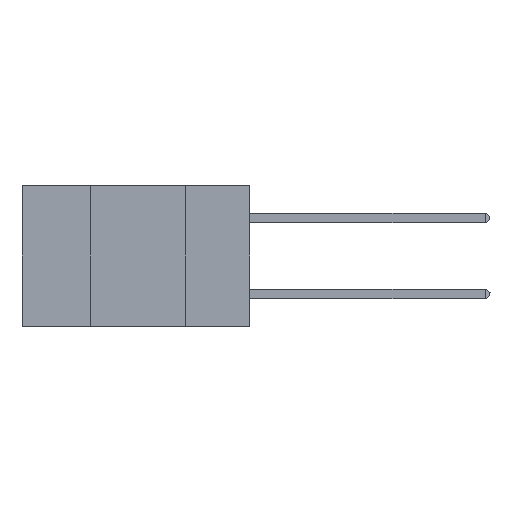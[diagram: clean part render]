
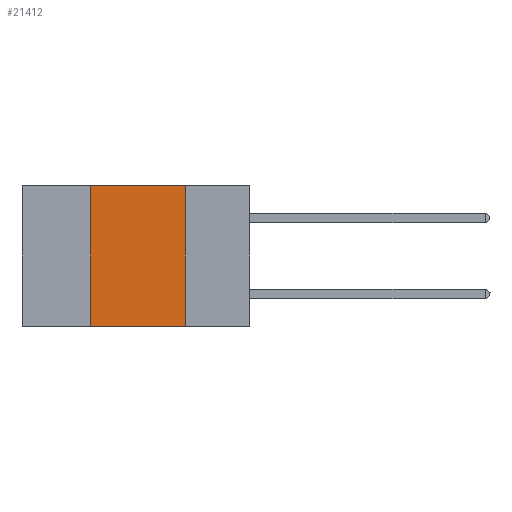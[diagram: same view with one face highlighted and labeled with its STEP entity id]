
A CAD part, left-side view. The second image highlights one B-rep face of the part: STEP entity #21412.
In plain terms, the highlighted planar face has unit normal (-1, 0, 0).
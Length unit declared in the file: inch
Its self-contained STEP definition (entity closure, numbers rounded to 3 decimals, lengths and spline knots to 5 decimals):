
#356 = CARTESIAN_POINT ( 'NONE',  ( 0., 0.17, 0. ) ) ;
#453 = DIRECTION ( 'NONE',  ( 0., 0., -1. ) ) ;
#1341 = CARTESIAN_POINT ( 'NONE',  ( 0., 0.17, -0.37 ) ) ;
#1901 = CARTESIAN_POINT ( 'NONE',  ( 0., 0.42, -0.37 ) ) ;
#3187 = VERTEX_POINT ( 'NONE', #1341 ) ;
#3577 = FACE_OUTER_BOUND ( 'NONE', #20841, .T. ) ;
#3789 = DIRECTION ( 'NONE',  ( 0., 0., 1. ) ) ;
#5451 = VERTEX_POINT ( 'NONE', #356 ) ;
#5716 = ORIENTED_EDGE ( 'NONE', *, *, #7045, .F. ) ;
#7045 = EDGE_CURVE ( 'NONE', #27275, #5451, #21480, .T. ) ;
#7298 = VECTOR ( 'NONE', #16778, 39.37008 ) ;
#8743 = AXIS2_PLACEMENT_3D ( 'NONE', #34308, #20629, #44646 ) ;
#13847 = EDGE_CURVE ( 'NONE', #37993, #3187, #17581, .T. ) ;
#16778 = DIRECTION ( 'NONE',  ( 0., -1., 0. ) ) ;
#17581 = LINE ( 'NONE', #33947, #7298 ) ;
#20629 = DIRECTION ( 'NONE',  ( 1., 0., 0. ) ) ;
#20841 = EDGE_LOOP ( 'NONE', ( #28211, #5716, #31731, #32651 ) ) ;
#21412 = ADVANCED_FACE ( 'NONE', ( #3577 ), #41209, .F. ) ;
#21480 = LINE ( 'NONE', #25908, #38646 ) ;
#22913 = VECTOR ( 'NONE', #3789, 39.37008 ) ;
#23172 = EDGE_CURVE ( 'NONE', #37993, #27275, #32014, .T. ) ;
#25908 = CARTESIAN_POINT ( 'NONE',  ( 0., 0.6, 0. ) ) ;
#27275 = VERTEX_POINT ( 'NONE', #39365 ) ;
#28211 = ORIENTED_EDGE ( 'NONE', *, *, #38377, .F. ) ;
#29316 = DIRECTION ( 'NONE',  ( 0., -1., 0. ) ) ;
#31731 = ORIENTED_EDGE ( 'NONE', *, *, #23172, .F. ) ;
#32014 = LINE ( 'NONE', #34762, #22913 ) ;
#32651 = ORIENTED_EDGE ( 'NONE', *, *, #13847, .T. ) ;
#33947 = CARTESIAN_POINT ( 'NONE',  ( 0., 0.6, -0.37 ) ) ;
#34308 = CARTESIAN_POINT ( 'NONE',  ( 0., 0.6, 0. ) ) ;
#34762 = CARTESIAN_POINT ( 'NONE',  ( 0., 0.42, 0. ) ) ;
#37993 = VERTEX_POINT ( 'NONE', #1901 ) ;
#38377 = EDGE_CURVE ( 'NONE', #5451, #3187, #43761, .T. ) ;
#38646 = VECTOR ( 'NONE', #29316, 39.37008 ) ;
#39365 = CARTESIAN_POINT ( 'NONE',  ( 0., 0.42, 0. ) ) ;
#41209 = PLANE ( 'NONE',  #8743 ) ;
#41843 = CARTESIAN_POINT ( 'NONE',  ( 0., 0.17, 0. ) ) ;
#42662 = VECTOR ( 'NONE', #453, 39.37008 ) ;
#43761 = LINE ( 'NONE', #41843, #42662 ) ;
#44646 = DIRECTION ( 'NONE',  ( 0., 0., -1. ) ) ;
